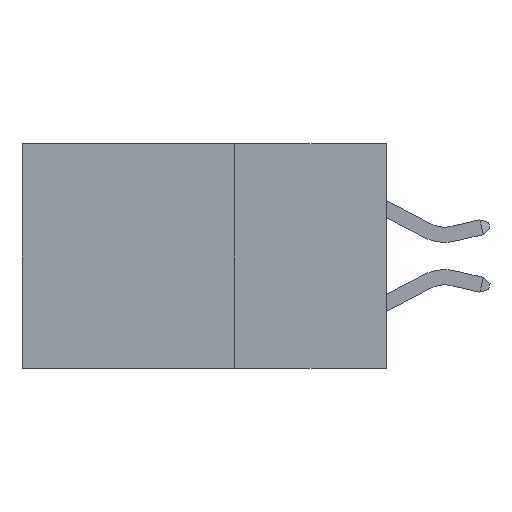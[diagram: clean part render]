
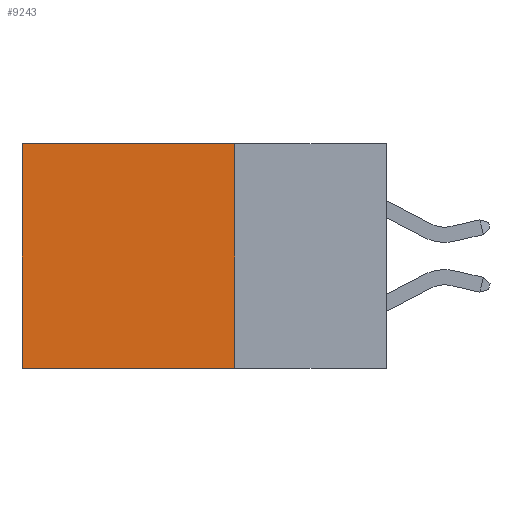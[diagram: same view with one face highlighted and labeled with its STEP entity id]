
A CAD part, left-side view. The second image highlights one B-rep face of the part: STEP entity #9243.
In plain terms, the highlighted planar face has unit normal (-1, 0, 0).
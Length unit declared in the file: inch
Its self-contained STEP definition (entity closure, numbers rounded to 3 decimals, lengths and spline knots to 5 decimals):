
#394 = EDGE_CURVE ( 'NONE', #6544, #1661, #3823, .T. ) ;
#595 = PLANE ( 'NONE',  #7270 ) ;
#717 = CARTESIAN_POINT ( 'NONE',  ( 0.2615, 0.25, -0.37 ) ) ;
#1637 = CARTESIAN_POINT ( 'NONE',  ( 0.2615, 0.25, -0.37 ) ) ;
#1661 = VERTEX_POINT ( 'NONE', #9131 ) ;
#1866 = EDGE_CURVE ( 'NONE', #5521, #1661, #4285, .T. ) ;
#1926 = EDGE_CURVE ( 'NONE', #9728, #6544, #4934, .T. ) ;
#2365 = FACE_OUTER_BOUND ( 'NONE', #3865, .T. ) ;
#2674 = DIRECTION ( 'NONE',  ( 1., 0., 0. ) ) ;
#2683 = ORIENTED_EDGE ( 'NONE', *, *, #1866, .T. ) ;
#2801 = CARTESIAN_POINT ( 'NONE',  ( 0.2615, 0.25, -0.37 ) ) ;
#3023 = DIRECTION ( 'NONE',  ( 0., 0., -1. ) ) ;
#3054 = CARTESIAN_POINT ( 'NONE',  ( 0.2615, 0.6, -0.37 ) ) ;
#3094 = CARTESIAN_POINT ( 'NONE',  ( 0.2615, 0.25, 0. ) ) ;
#3821 = CARTESIAN_POINT ( 'NONE',  ( 0.2615, 0.6, 0. ) ) ;
#3823 = LINE ( 'NONE', #717, #8354 ) ;
#3865 = EDGE_LOOP ( 'NONE', ( #2683, #11319, #8044, #5764 ) ) ;
#4158 = VECTOR ( 'NONE', #5736, 39.37008 ) ;
#4285 = LINE ( 'NONE', #3054, #8271 ) ;
#4934 = LINE ( 'NONE', #8798, #9173 ) ;
#5521 = VERTEX_POINT ( 'NONE', #3821 ) ;
#5736 = DIRECTION ( 'NONE',  ( 0., 1., 0. ) ) ;
#5764 = ORIENTED_EDGE ( 'NONE', *, *, #9010, .T. ) ;
#6434 = LINE ( 'NONE', #3094, #4158 ) ;
#6544 = VERTEX_POINT ( 'NONE', #2801 ) ;
#7270 = AXIS2_PLACEMENT_3D ( 'NONE', #1637, #2674, #8723 ) ;
#8044 = ORIENTED_EDGE ( 'NONE', *, *, #1926, .F. ) ;
#8271 = VECTOR ( 'NONE', #3023, 39.37008 ) ;
#8354 = VECTOR ( 'NONE', #9662, 39.37008 ) ;
#8723 = DIRECTION ( 'NONE',  ( 0., 0., -1. ) ) ;
#8798 = CARTESIAN_POINT ( 'NONE',  ( 0.2615, 0.25, -0.37 ) ) ;
#8834 = DIRECTION ( 'NONE',  ( 0., 0., -1. ) ) ;
#9010 = EDGE_CURVE ( 'NONE', #9728, #5521, #6434, .T. ) ;
#9131 = CARTESIAN_POINT ( 'NONE',  ( 0.2615, 0.6, -0.37 ) ) ;
#9157 = CARTESIAN_POINT ( 'NONE',  ( 0.2615, 0.25, 0. ) ) ;
#9173 = VECTOR ( 'NONE', #8834, 39.37008 ) ;
#9243 = ADVANCED_FACE ( 'NONE', ( #2365 ), #595, .F. ) ;
#9662 = DIRECTION ( 'NONE',  ( 0., 1., 0. ) ) ;
#9728 = VERTEX_POINT ( 'NONE', #9157 ) ;
#11319 = ORIENTED_EDGE ( 'NONE', *, *, #394, .F. ) ;
